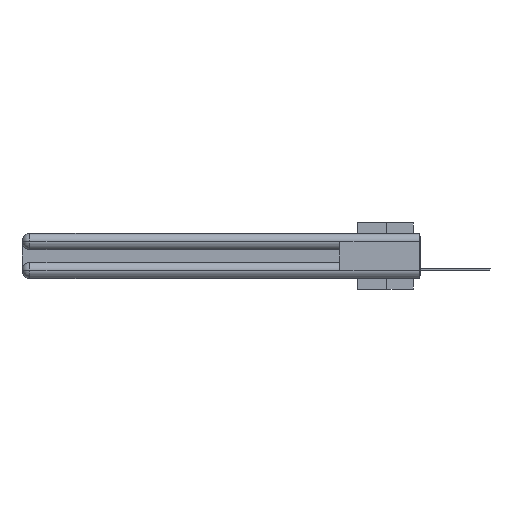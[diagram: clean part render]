
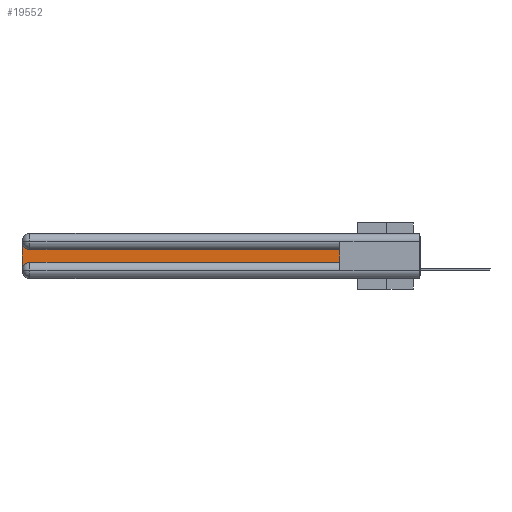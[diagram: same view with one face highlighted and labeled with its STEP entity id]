
A CAD part, left-side view. The second image highlights one B-rep face of the part: STEP entity #19552.
In plain terms, the highlighted planar face has unit normal (-1, 0, 0).
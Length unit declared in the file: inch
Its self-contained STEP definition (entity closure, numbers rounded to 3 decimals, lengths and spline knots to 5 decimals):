
#1957 = ORIENTED_EDGE ( 'NONE', *, *, #19675, .T. ) ;
#2104 = CARTESIAN_POINT ( 'NONE',  ( 0.075, 0.6, -0.1225 ) ) ;
#2398 = CARTESIAN_POINT ( 'NONE',  ( 0.075, 2.94, -0.1225 ) ) ;
#3989 = AXIS2_PLACEMENT_3D ( 'NONE', #28654, #5927, #31204 ) ;
#4728 = VECTOR ( 'NONE', #24864, 39.37008 ) ;
#5135 = VERTEX_POINT ( 'NONE', #29482 ) ;
#5444 = EDGE_CURVE ( 'NONE', #17197, #19157, #26641, .T. ) ;
#5879 = EDGE_CURVE ( 'NONE', #19157, #5135, #27403, .T. ) ;
#5927 = DIRECTION ( 'NONE',  ( 1., 0., 0. ) ) ;
#6322 = ORIENTED_EDGE ( 'NONE', *, *, #5879, .T. ) ;
#6638 = CARTESIAN_POINT ( 'NONE',  ( 0.075, 3., -0.2775 ) ) ;
#6684 = DIRECTION ( 'NONE',  ( 0., 0., -1. ) ) ;
#6791 = FACE_OUTER_BOUND ( 'NONE', #18461, .T. ) ;
#7268 = CARTESIAN_POINT ( 'NONE',  ( 0.075, 0.6, -0.2175 ) ) ;
#7343 = DIRECTION ( 'NONE',  ( 1., 0., 0. ) ) ;
#7767 = VERTEX_POINT ( 'NONE', #6638 ) ;
#8453 = VERTEX_POINT ( 'NONE', #19430 ) ;
#9295 = ORIENTED_EDGE ( 'NONE', *, *, #30985, .T. ) ;
#9583 = LINE ( 'NONE', #15382, #11128 ) ;
#9991 = CARTESIAN_POINT ( 'NONE',  ( 0.075, 2.94, -0.2175 ) ) ;
#10229 = EDGE_CURVE ( 'NONE', #5135, #12043, #11446, .T. ) ;
#11128 = VECTOR ( 'NONE', #12942, 39.37008 ) ;
#11440 = ORIENTED_EDGE ( 'NONE', *, *, #5444, .T. ) ;
#11446 = LINE ( 'NONE', #2104, #4728 ) ;
#12043 = VERTEX_POINT ( 'NONE', #2398 ) ;
#12942 = DIRECTION ( 'NONE',  ( 0., 0., -1. ) ) ;
#14760 = CARTESIAN_POINT ( 'NONE',  ( 0.075, 2.94, -0.0625 ) ) ;
#15382 = CARTESIAN_POINT ( 'NONE',  ( 0.075, 3., -0.2175 ) ) ;
#17197 = VERTEX_POINT ( 'NONE', #9991 ) ;
#17665 = DIRECTION ( 'NONE',  ( 0., 0., 1. ) ) ;
#18244 = CIRCLE ( 'NONE', #3989, 0.06 ) ;
#18461 = EDGE_LOOP ( 'NONE', ( #32736, #1957, #9295, #25205, #11440, #6322 ) ) ;
#19157 = VERTEX_POINT ( 'NONE', #7268 ) ;
#19430 = CARTESIAN_POINT ( 'NONE',  ( 0.075, 3., -0.0625 ) ) ;
#19552 = ADVANCED_FACE ( 'NONE', ( #6791 ), #23568, .F. ) ;
#19675 = EDGE_CURVE ( 'NONE', #12043, #8453, #27710, .T. ) ;
#20223 = DIRECTION ( 'NONE',  ( 0., -1., 0. ) ) ;
#20665 = EDGE_CURVE ( 'NONE', #7767, #17197, #18244, .T. ) ;
#20692 = VECTOR ( 'NONE', #17665, 39.37008 ) ;
#21116 = AXIS2_PLACEMENT_3D ( 'NONE', #14760, #7343, #27203 ) ;
#23568 = PLANE ( 'NONE',  #30808 ) ;
#24864 = DIRECTION ( 'NONE',  ( 0., 1., 0. ) ) ;
#25205 = ORIENTED_EDGE ( 'NONE', *, *, #20665, .T. ) ;
#26211 = CARTESIAN_POINT ( 'NONE',  ( 0.075, 3., -0.1225 ) ) ;
#26641 = LINE ( 'NONE', #28014, #29799 ) ;
#27203 = DIRECTION ( 'NONE',  ( 0., 0., -1. ) ) ;
#27403 = LINE ( 'NONE', #32112, #20692 ) ;
#27710 = CIRCLE ( 'NONE', #21116, 0.06 ) ;
#28014 = CARTESIAN_POINT ( 'NONE',  ( 0.075, 0.6, -0.2175 ) ) ;
#28654 = CARTESIAN_POINT ( 'NONE',  ( 0.075, 2.94, -0.2775 ) ) ;
#29482 = CARTESIAN_POINT ( 'NONE',  ( 0.075, 0.6, -0.1225 ) ) ;
#29799 = VECTOR ( 'NONE', #20223, 39.37008 ) ;
#30808 = AXIS2_PLACEMENT_3D ( 'NONE', #26211, #31614, #6684 ) ;
#30985 = EDGE_CURVE ( 'NONE', #8453, #7767, #9583, .T. ) ;
#31204 = DIRECTION ( 'NONE',  ( 0., 0., -1. ) ) ;
#31614 = DIRECTION ( 'NONE',  ( 1., 0., 0. ) ) ;
#32112 = CARTESIAN_POINT ( 'NONE',  ( 0.075, 0.6, -0.2175 ) ) ;
#32736 = ORIENTED_EDGE ( 'NONE', *, *, #10229, .T. ) ;
